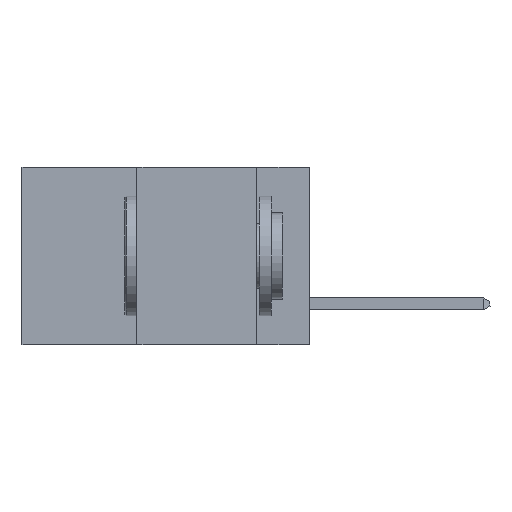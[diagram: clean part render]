
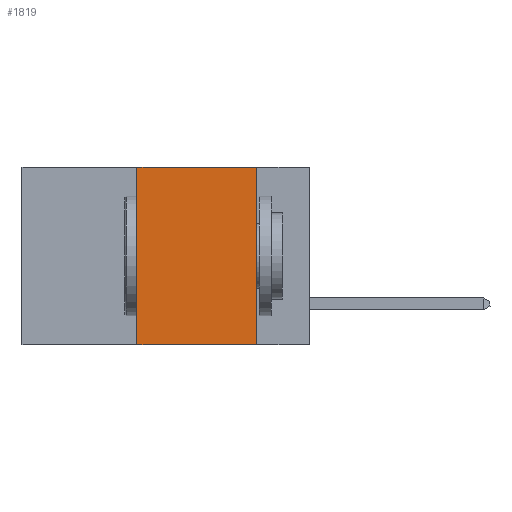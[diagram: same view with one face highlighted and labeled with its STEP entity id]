
A CAD part, left-side view. The second image highlights one B-rep face of the part: STEP entity #1819.
In plain terms, the highlighted planar face has unit normal (-1, 0, 0).
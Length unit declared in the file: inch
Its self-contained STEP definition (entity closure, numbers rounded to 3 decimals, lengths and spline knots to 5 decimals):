
#55 = DIRECTION ( 'NONE',  ( 0., 0., -1. ) ) ;
#81 = DIRECTION ( 'NONE',  ( 0., -1., 0. ) ) ;
#457 = ORIENTED_EDGE ( 'NONE', *, *, #1949, .F. ) ;
#511 = DIRECTION ( 'NONE',  ( 0., -1., 0. ) ) ;
#778 = CARTESIAN_POINT ( 'NONE',  ( 0., 0.36, 0. ) ) ;
#1028 = VECTOR ( 'NONE', #4304, 39.37008 ) ;
#1094 = ORIENTED_EDGE ( 'NONE', *, *, #3112, .T. ) ;
#1357 = LINE ( 'NONE', #7966, #1028 ) ;
#1501 = CARTESIAN_POINT ( 'NONE',  ( 0., 0.6, 0. ) ) ;
#1562 = EDGE_CURVE ( 'NONE', #1808, #6873, #1357, .T. ) ;
#1587 = LINE ( 'NONE', #1501, #3330 ) ;
#1808 = VERTEX_POINT ( 'NONE', #4338 ) ;
#1819 = ADVANCED_FACE ( 'NONE', ( #4971 ), #2925, .F. ) ;
#1949 = EDGE_CURVE ( 'NONE', #6873, #8837, #1587, .T. ) ;
#2176 = DIRECTION ( 'NONE',  ( 1., 0., 0. ) ) ;
#2240 = VECTOR ( 'NONE', #511, 39.37008 ) ;
#2495 = EDGE_LOOP ( 'NONE', ( #3750, #457, #4458, #1094 ) ) ;
#2742 = EDGE_CURVE ( 'NONE', #8837, #4558, #4820, .T. ) ;
#2925 = PLANE ( 'NONE',  #5602 ) ;
#2931 = CARTESIAN_POINT ( 'NONE',  ( 0., 0.11, 0. ) ) ;
#3112 = EDGE_CURVE ( 'NONE', #1808, #4558, #6186, .T. ) ;
#3330 = VECTOR ( 'NONE', #81, 39.37008 ) ;
#3684 = DIRECTION ( 'NONE',  ( 0., 0., -1. ) ) ;
#3750 = ORIENTED_EDGE ( 'NONE', *, *, #2742, .F. ) ;
#4304 = DIRECTION ( 'NONE',  ( 0., 0., 1. ) ) ;
#4338 = CARTESIAN_POINT ( 'NONE',  ( 0., 0.36, -0.37 ) ) ;
#4458 = ORIENTED_EDGE ( 'NONE', *, *, #1562, .F. ) ;
#4479 = VECTOR ( 'NONE', #55, 39.37008 ) ;
#4558 = VERTEX_POINT ( 'NONE', #6077 ) ;
#4820 = LINE ( 'NONE', #2931, #4479 ) ;
#4954 = CARTESIAN_POINT ( 'NONE',  ( 0., 0.6, -0.37 ) ) ;
#4971 = FACE_OUTER_BOUND ( 'NONE', #2495, .T. ) ;
#5157 = CARTESIAN_POINT ( 'NONE',  ( 0., 0.6, 0. ) ) ;
#5602 = AXIS2_PLACEMENT_3D ( 'NONE', #5157, #2176, #3684 ) ;
#6077 = CARTESIAN_POINT ( 'NONE',  ( 0., 0.11, -0.37 ) ) ;
#6186 = LINE ( 'NONE', #4954, #2240 ) ;
#6873 = VERTEX_POINT ( 'NONE', #778 ) ;
#7966 = CARTESIAN_POINT ( 'NONE',  ( 0., 0.36, 0. ) ) ;
#8820 = CARTESIAN_POINT ( 'NONE',  ( 0., 0.11, 0. ) ) ;
#8837 = VERTEX_POINT ( 'NONE', #8820 ) ;
